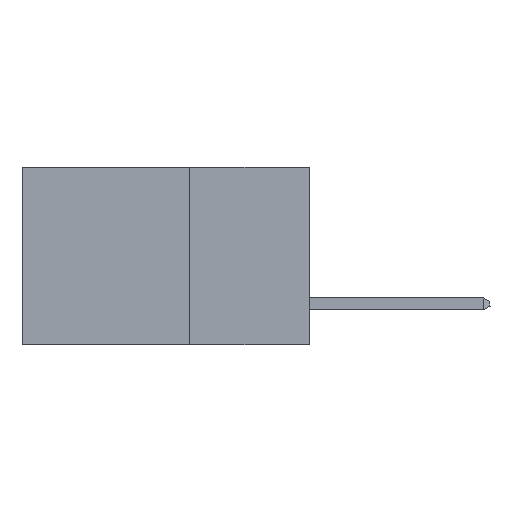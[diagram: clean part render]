
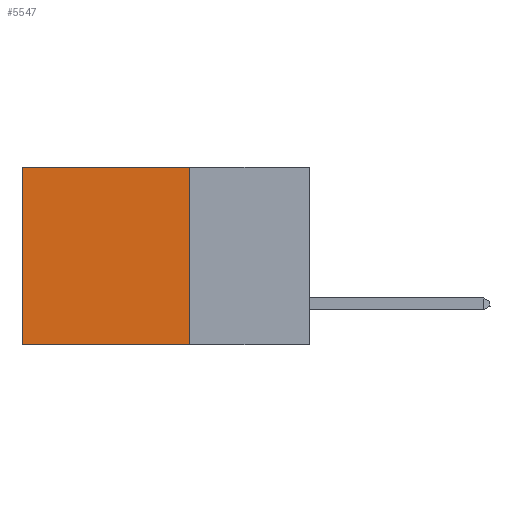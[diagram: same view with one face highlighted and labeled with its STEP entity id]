
A CAD part, left-side view. The second image highlights one B-rep face of the part: STEP entity #5547.
In plain terms, the highlighted planar face has unit normal (-1, 0, 0).
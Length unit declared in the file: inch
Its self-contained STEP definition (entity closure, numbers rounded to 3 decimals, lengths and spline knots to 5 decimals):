
#293 = DIRECTION ( 'NONE',  ( 0., 1., 0. ) ) ;
#556 = CARTESIAN_POINT ( 'NONE',  ( 0.2875, 0.25, -0.37 ) ) ;
#613 = CARTESIAN_POINT ( 'NONE',  ( 0.2875, 0.25, 0. ) ) ;
#1064 = ORIENTED_EDGE ( 'NONE', *, *, #1487, .F. ) ;
#1245 = CARTESIAN_POINT ( 'NONE',  ( 0.2875, 0.6, 0. ) ) ;
#1487 = EDGE_CURVE ( 'NONE', #3425, #5001, #15613, .T. ) ;
#1640 = VERTEX_POINT ( 'NONE', #6665 ) ;
#2685 = CARTESIAN_POINT ( 'NONE',  ( 0.2875, 0.25, 0. ) ) ;
#3425 = VERTEX_POINT ( 'NONE', #2685 ) ;
#3433 = VECTOR ( 'NONE', #293, 39.37008 ) ;
#4022 = VECTOR ( 'NONE', #7248, 39.37008 ) ;
#4332 = EDGE_CURVE ( 'NONE', #3425, #18314, #7359, .T. ) ;
#4356 = PLANE ( 'NONE',  #8946 ) ;
#4849 = ORIENTED_EDGE ( 'NONE', *, *, #4332, .T. ) ;
#4962 = VECTOR ( 'NONE', #11050, 39.37008 ) ;
#5001 = VERTEX_POINT ( 'NONE', #9052 ) ;
#5532 = EDGE_CURVE ( 'NONE', #18314, #1640, #7937, .T. ) ;
#5547 = ADVANCED_FACE ( 'NONE', ( #11911 ), #4356, .F. ) ;
#5849 = DIRECTION ( 'NONE',  ( 0., 0., -1. ) ) ;
#5893 = LINE ( 'NONE', #556, #4962 ) ;
#6665 = CARTESIAN_POINT ( 'NONE',  ( 0.2875, 0.6, -0.37 ) ) ;
#7248 = DIRECTION ( 'NONE',  ( 0., 0., -1. ) ) ;
#7268 = CARTESIAN_POINT ( 'NONE',  ( 0.2875, 0.6, 0. ) ) ;
#7359 = LINE ( 'NONE', #613, #3433 ) ;
#7550 = ORIENTED_EDGE ( 'NONE', *, *, #5532, .T. ) ;
#7707 = VECTOR ( 'NONE', #11267, 39.37008 ) ;
#7937 = LINE ( 'NONE', #1245, #4022 ) ;
#8027 = EDGE_LOOP ( 'NONE', ( #7550, #11956, #1064, #4849 ) ) ;
#8946 = AXIS2_PLACEMENT_3D ( 'NONE', #11760, #19074, #5849 ) ;
#9052 = CARTESIAN_POINT ( 'NONE',  ( 0.2875, 0.25, -0.37 ) ) ;
#11050 = DIRECTION ( 'NONE',  ( 0., 1., 0. ) ) ;
#11267 = DIRECTION ( 'NONE',  ( 0., 0., -1. ) ) ;
#11370 = CARTESIAN_POINT ( 'NONE',  ( 0.2875, 0.25, 0. ) ) ;
#11760 = CARTESIAN_POINT ( 'NONE',  ( 0.2875, 0.25, 0. ) ) ;
#11911 = FACE_OUTER_BOUND ( 'NONE', #8027, .T. ) ;
#11956 = ORIENTED_EDGE ( 'NONE', *, *, #15320, .F. ) ;
#15320 = EDGE_CURVE ( 'NONE', #5001, #1640, #5893, .T. ) ;
#15613 = LINE ( 'NONE', #11370, #7707 ) ;
#18314 = VERTEX_POINT ( 'NONE', #7268 ) ;
#19074 = DIRECTION ( 'NONE',  ( 1., 0., 0. ) ) ;
